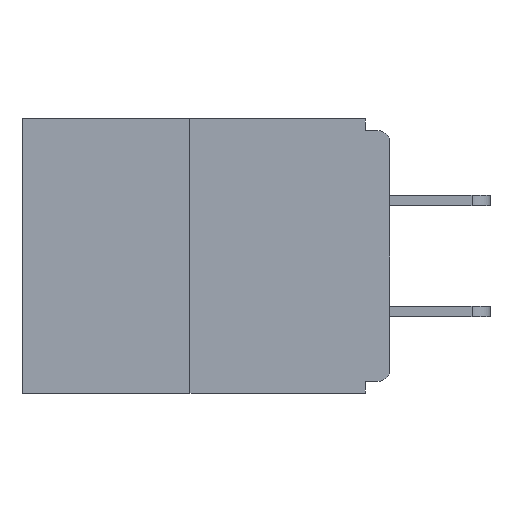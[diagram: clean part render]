
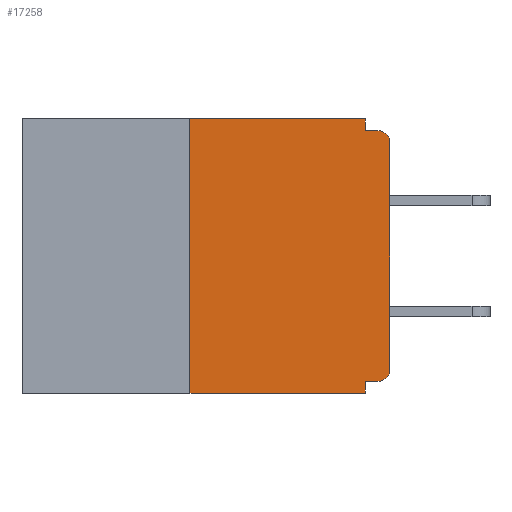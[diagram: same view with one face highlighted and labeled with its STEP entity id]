
A CAD part, left-side view. The second image highlights one B-rep face of the part: STEP entity #17258.
In plain terms, the highlighted planar face has unit normal (-1, 0, 0).
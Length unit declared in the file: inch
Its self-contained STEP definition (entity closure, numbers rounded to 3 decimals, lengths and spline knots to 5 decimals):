
#17 = VECTOR ( 'NONE', #10080, 39.37008 ) ;
#40 = VECTOR ( 'NONE', #15792, 39.37008 ) ;
#473 = EDGE_CURVE ( 'NONE', #14061, #3179, #8442, .T. ) ;
#548 = AXIS2_PLACEMENT_3D ( 'NONE', #20320, #15340, #15486 ) ;
#706 = EDGE_CURVE ( 'NONE', #8453, #4349, #5074, .T. ) ;
#1967 = DIRECTION ( 'NONE',  ( 0., 0., -1. ) ) ;
#2143 = CARTESIAN_POINT ( 'NONE',  ( 0., 0., -0.313 ) ) ;
#2462 = ORIENTED_EDGE ( 'NONE', *, *, #10929, .T. ) ;
#2485 = ORIENTED_EDGE ( 'NONE', *, *, #12200, .F. ) ;
#2500 = PLANE ( 'NONE',  #3512 ) ;
#2512 = ORIENTED_EDGE ( 'NONE', *, *, #14796, .F. ) ;
#2796 = AXIS2_PLACEMENT_3D ( 'NONE', #6696, #6764, #1967 ) ;
#2953 = VERTEX_POINT ( 'NONE', #17642 ) ;
#3179 = VERTEX_POINT ( 'NONE', #13139 ) ;
#3202 = CARTESIAN_POINT ( 'NONE',  ( 0., 0., 0. ) ) ;
#3358 = LINE ( 'NONE', #10959, #4409 ) ;
#3452 = CARTESIAN_POINT ( 'NONE',  ( 0., 0.015, -0.015 ) ) ;
#3512 = AXIS2_PLACEMENT_3D ( 'NONE', #7509, #14255, #15925 ) ;
#3760 = ORIENTED_EDGE ( 'NONE', *, *, #473, .F. ) ;
#4349 = VERTEX_POINT ( 'NONE', #18893 ) ;
#4409 = VECTOR ( 'NONE', #14219, 39.37008 ) ;
#4438 = FACE_OUTER_BOUND ( 'NONE', #4703, .T. ) ;
#4614 = VERTEX_POINT ( 'NONE', #8106 ) ;
#4703 = EDGE_LOOP ( 'NONE', ( #21415, #13832, #2462, #2512, #13143, #9300, #6978, #6740, #2485, #3760 ) ) ;
#4899 = LINE ( 'NONE', #17342, #8280 ) ;
#5074 = LINE ( 'NONE', #17256, #7683 ) ;
#6176 = DIRECTION ( 'NONE',  ( 0., 0., -1. ) ) ;
#6484 = EDGE_CURVE ( 'NONE', #6732, #2953, #10897, .T. ) ;
#6696 = CARTESIAN_POINT ( 'NONE',  ( 0., 0.015, -0.313 ) ) ;
#6732 = VERTEX_POINT ( 'NONE', #2143 ) ;
#6740 = ORIENTED_EDGE ( 'NONE', *, *, #21188, .T. ) ;
#6764 = DIRECTION ( 'NONE',  ( -1., 0., 0. ) ) ;
#6978 = ORIENTED_EDGE ( 'NONE', *, *, #6484, .T. ) ;
#6994 = EDGE_CURVE ( 'NONE', #4614, #9370, #3358, .T. ) ;
#7303 = LINE ( 'NONE', #14050, #40 ) ;
#7509 = CARTESIAN_POINT ( 'NONE',  ( 0., 0.46, 0. ) ) ;
#7683 = VECTOR ( 'NONE', #20633, 39.37008 ) ;
#8080 = CIRCLE ( 'NONE', #548, 0.015 ) ;
#8106 = CARTESIAN_POINT ( 'NONE',  ( 0., 0.015, -0.328 ) ) ;
#8199 = VECTOR ( 'NONE', #6176, 39.37008 ) ;
#8280 = VECTOR ( 'NONE', #19206, 39.37008 ) ;
#8442 = LINE ( 'NONE', #21158, #8199 ) ;
#8453 = VERTEX_POINT ( 'NONE', #20927 ) ;
#8491 = CARTESIAN_POINT ( 'NONE',  ( 0., 0.46, -0.343 ) ) ;
#8696 = VERTEX_POINT ( 'NONE', #3452 ) ;
#9159 = CIRCLE ( 'NONE', #2796, 0.015 ) ;
#9300 = ORIENTED_EDGE ( 'NONE', *, *, #14744, .T. ) ;
#9370 = VERTEX_POINT ( 'NONE', #15892 ) ;
#10080 = DIRECTION ( 'NONE',  ( 0., -1., 0. ) ) ;
#10701 = EDGE_CURVE ( 'NONE', #4349, #14061, #7303, .T. ) ;
#10897 = LINE ( 'NONE', #3202, #20811 ) ;
#10929 = EDGE_CURVE ( 'NONE', #8453, #11509, #10953, .T. ) ;
#10953 = LINE ( 'NONE', #8491, #17 ) ;
#10959 = CARTESIAN_POINT ( 'NONE',  ( 0., 0., -0.328 ) ) ;
#11471 = DIRECTION ( 'NONE',  ( 0., 0., 1. ) ) ;
#11509 = VERTEX_POINT ( 'NONE', #17696 ) ;
#11849 = DIRECTION ( 'NONE',  ( 0., 0., -1. ) ) ;
#12200 = EDGE_CURVE ( 'NONE', #3179, #8696, #4899, .T. ) ;
#13139 = CARTESIAN_POINT ( 'NONE',  ( 0., 0.031, -0.015 ) ) ;
#13143 = ORIENTED_EDGE ( 'NONE', *, *, #6994, .F. ) ;
#13832 = ORIENTED_EDGE ( 'NONE', *, *, #706, .F. ) ;
#14050 = CARTESIAN_POINT ( 'NONE',  ( 0., 0.46, 0. ) ) ;
#14061 = VERTEX_POINT ( 'NONE', #17614 ) ;
#14219 = DIRECTION ( 'NONE',  ( 0., 1., 0. ) ) ;
#14255 = DIRECTION ( 'NONE',  ( 1., 0., 0. ) ) ;
#14744 = EDGE_CURVE ( 'NONE', #4614, #6732, #9159, .T. ) ;
#14796 = EDGE_CURVE ( 'NONE', #9370, #11509, #20634, .T. ) ;
#15340 = DIRECTION ( 'NONE',  ( -1., 0., 0. ) ) ;
#15486 = DIRECTION ( 'NONE',  ( 0., 0., -1. ) ) ;
#15792 = DIRECTION ( 'NONE',  ( 0., -1., 0. ) ) ;
#15892 = CARTESIAN_POINT ( 'NONE',  ( 0., 0.031, -0.328 ) ) ;
#15925 = DIRECTION ( 'NONE',  ( 0., 0., -1. ) ) ;
#16706 = CARTESIAN_POINT ( 'NONE',  ( 0., 0.031, -0.343 ) ) ;
#17256 = CARTESIAN_POINT ( 'NONE',  ( 0., 0.25, 0. ) ) ;
#17258 = ADVANCED_FACE ( 'NONE', ( #4438 ), #2500, .F. ) ;
#17342 = CARTESIAN_POINT ( 'NONE',  ( 0., 0., -0.015 ) ) ;
#17614 = CARTESIAN_POINT ( 'NONE',  ( 0., 0.031, 0. ) ) ;
#17642 = CARTESIAN_POINT ( 'NONE',  ( 0., 0., -0.03 ) ) ;
#17696 = CARTESIAN_POINT ( 'NONE',  ( 0., 0.031, -0.343 ) ) ;
#18893 = CARTESIAN_POINT ( 'NONE',  ( 0., 0.25, 0. ) ) ;
#19206 = DIRECTION ( 'NONE',  ( 0., -1., 0. ) ) ;
#20320 = CARTESIAN_POINT ( 'NONE',  ( 0., 0.015, -0.03 ) ) ;
#20358 = VECTOR ( 'NONE', #11849, 39.37008 ) ;
#20633 = DIRECTION ( 'NONE',  ( 0., 0., 1. ) ) ;
#20634 = LINE ( 'NONE', #16706, #20358 ) ;
#20811 = VECTOR ( 'NONE', #11471, 39.37008 ) ;
#20927 = CARTESIAN_POINT ( 'NONE',  ( 0., 0.25, -0.343 ) ) ;
#21158 = CARTESIAN_POINT ( 'NONE',  ( 0., 0.031, 0. ) ) ;
#21188 = EDGE_CURVE ( 'NONE', #2953, #8696, #8080, .T. ) ;
#21415 = ORIENTED_EDGE ( 'NONE', *, *, #10701, .F. ) ;
